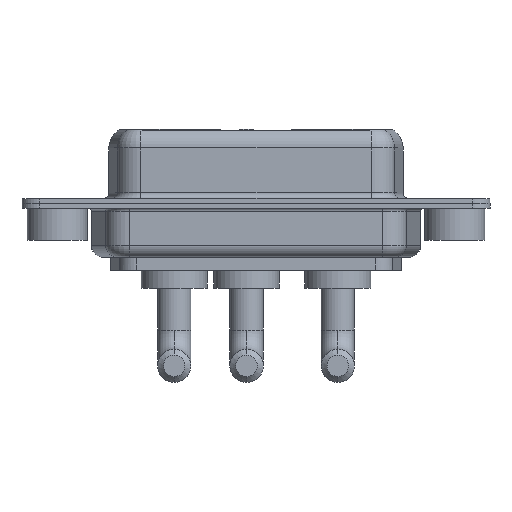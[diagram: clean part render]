
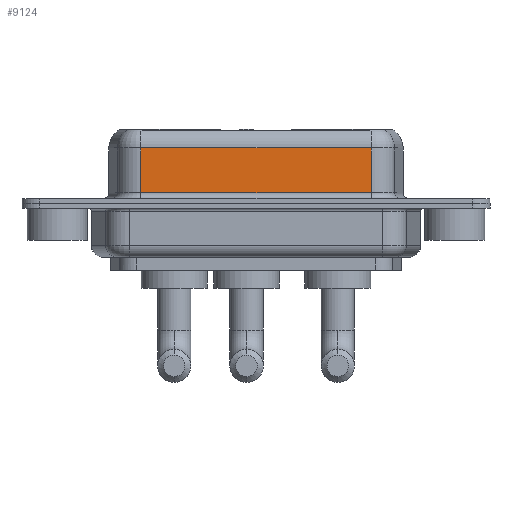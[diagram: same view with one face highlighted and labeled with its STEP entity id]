
A CAD part, front view. The second image highlights one B-rep face of the part: STEP entity #9124.
In plain terms, the highlighted planar face has unit normal (0, -1, 0).
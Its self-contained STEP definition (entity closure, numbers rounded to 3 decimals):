
#192 = VECTOR ( 'NONE', #12403, 1000. ) ;
#1129 = AXIS2_PLACEMENT_3D ( 'NONE', #2539, #2749, #1900 ) ;
#1287 = LINE ( 'NONE', #10949, #13369 ) ;
#1874 = EDGE_CURVE ( 'NONE', #10589, #12569, #1287, .T. ) ;
#1900 = DIRECTION ( 'NONE',  ( 0., 0., 1. ) ) ;
#2539 = CARTESIAN_POINT ( 'NONE',  ( 26.287, -3.95, 6.4 ) ) ;
#2749 = DIRECTION ( 'NONE',  ( 0., 1., 0. ) ) ;
#3133 = VECTOR ( 'NONE', #5785, 1000. ) ;
#3579 = PLANE ( 'NONE',  #1129 ) ;
#3628 = ORIENTED_EDGE ( 'NONE', *, *, #1874, .T. ) ;
#3874 = ORIENTED_EDGE ( 'NONE', *, *, #5117, .F. ) ;
#3936 = VECTOR ( 'NONE', #5568, 1000. ) ;
#5117 = EDGE_CURVE ( 'NONE', #10589, #12541, #5992, .T. ) ;
#5568 = DIRECTION ( 'NONE',  ( 1., 0., 0. ) ) ;
#5785 = DIRECTION ( 'NONE',  ( 0., 0., -1. ) ) ;
#5890 = CARTESIAN_POINT ( 'NONE',  ( 7.013, -3.95, 6.4 ) ) ;
#5992 = LINE ( 'NONE', #8116, #3133 ) ;
#6740 = EDGE_CURVE ( 'NONE', #9034, #12541, #6787, .T. ) ;
#6787 = LINE ( 'NONE', #8040, #3936 ) ;
#7158 = LINE ( 'NONE', #5890, #192 ) ;
#7817 = EDGE_CURVE ( 'NONE', #12569, #9034, #7158, .T. ) ;
#8040 = CARTESIAN_POINT ( 'NONE',  ( 26.287, -3.95, 0.9 ) ) ;
#8116 = CARTESIAN_POINT ( 'NONE',  ( 26.287, -3.95, 6.4 ) ) ;
#8235 = CARTESIAN_POINT ( 'NONE',  ( 26.287, -3.95, 0.9 ) ) ;
#8745 = CARTESIAN_POINT ( 'NONE',  ( 26.287, -3.95, 4.65 ) ) ;
#9007 = CARTESIAN_POINT ( 'NONE',  ( 7.013, -3.95, 4.65 ) ) ;
#9034 = VERTEX_POINT ( 'NONE', #12196 ) ;
#9124 = ADVANCED_FACE ( 'NONE', ( #9818 ), #3579, .F. ) ;
#9818 = FACE_OUTER_BOUND ( 'NONE', #11483, .T. ) ;
#10589 = VERTEX_POINT ( 'NONE', #8745 ) ;
#10817 = DIRECTION ( 'NONE',  ( -1., 0., 0. ) ) ;
#10949 = CARTESIAN_POINT ( 'NONE',  ( 26.287, -3.95, 4.65 ) ) ;
#11483 = EDGE_LOOP ( 'NONE', ( #3874, #3628, #11532, #12751 ) ) ;
#11532 = ORIENTED_EDGE ( 'NONE', *, *, #7817, .T. ) ;
#12196 = CARTESIAN_POINT ( 'NONE',  ( 7.013, -3.95, 0.9 ) ) ;
#12403 = DIRECTION ( 'NONE',  ( 0., 0., -1. ) ) ;
#12541 = VERTEX_POINT ( 'NONE', #8235 ) ;
#12569 = VERTEX_POINT ( 'NONE', #9007 ) ;
#12751 = ORIENTED_EDGE ( 'NONE', *, *, #6740, .T. ) ;
#13369 = VECTOR ( 'NONE', #10817, 1000. ) ;
